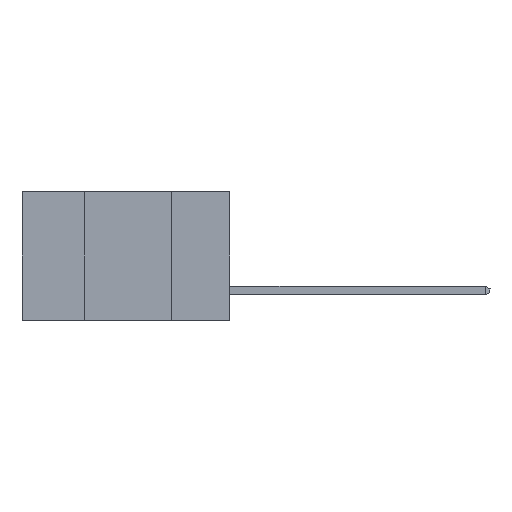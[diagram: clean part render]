
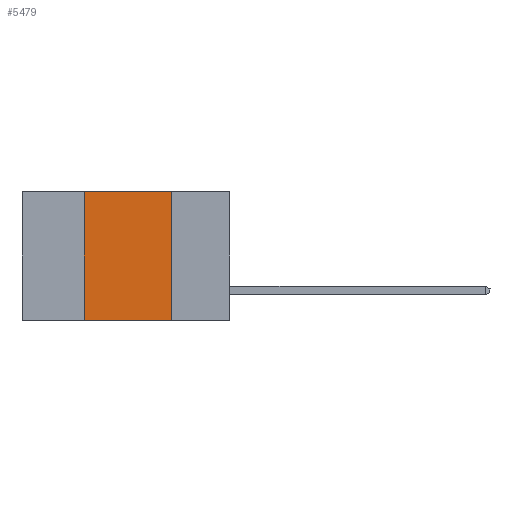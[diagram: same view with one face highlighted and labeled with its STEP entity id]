
A CAD part, left-side view. The second image highlights one B-rep face of the part: STEP entity #5479.
In plain terms, the highlighted planar face has unit normal (-1, 0, 0).
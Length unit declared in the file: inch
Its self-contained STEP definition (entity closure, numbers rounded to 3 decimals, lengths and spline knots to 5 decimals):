
#651 = VECTOR ( 'NONE', #3006, 39.37008 ) ;
#1235 = DIRECTION ( 'NONE',  ( 0., 0., -1. ) ) ;
#2057 = LINE ( 'NONE', #6154, #7532 ) ;
#2148 = DIRECTION ( 'NONE',  ( 0., 0., 1. ) ) ;
#2306 = CARTESIAN_POINT ( 'NONE',  ( 0., 0.42, -0.37 ) ) ;
#2531 = VERTEX_POINT ( 'NONE', #6071 ) ;
#2914 = CARTESIAN_POINT ( 'NONE',  ( 0., 0.17, -0.37 ) ) ;
#3006 = DIRECTION ( 'NONE',  ( 0., -1., 0. ) ) ;
#3350 = EDGE_CURVE ( 'NONE', #2531, #11595, #14398, .T. ) ;
#3627 = VECTOR ( 'NONE', #1235, 39.37008 ) ;
#4498 = VERTEX_POINT ( 'NONE', #2914 ) ;
#4834 = ORIENTED_EDGE ( 'NONE', *, *, #17452, .F. ) ;
#5479 = ADVANCED_FACE ( 'NONE', ( #7784 ), #17388, .F. ) ;
#6071 = CARTESIAN_POINT ( 'NONE',  ( 0., 0.42, 0. ) ) ;
#6154 = CARTESIAN_POINT ( 'NONE',  ( 0., 0.42, -0.37 ) ) ;
#6203 = DIRECTION ( 'NONE',  ( 1., 0., 0. ) ) ;
#6803 = ORIENTED_EDGE ( 'NONE', *, *, #15710, .T. ) ;
#6811 = AXIS2_PLACEMENT_3D ( 'NONE', #10497, #6203, #7614 ) ;
#7071 = EDGE_LOOP ( 'NONE', ( #17323, #12047, #4834, #6803 ) ) ;
#7104 = LINE ( 'NONE', #15414, #3627 ) ;
#7284 = EDGE_CURVE ( 'NONE', #11595, #4498, #7104, .T. ) ;
#7290 = CARTESIAN_POINT ( 'NONE',  ( 0., 0.6, -0.37 ) ) ;
#7532 = VECTOR ( 'NONE', #2148, 39.37008 ) ;
#7614 = DIRECTION ( 'NONE',  ( 0., 0., -1. ) ) ;
#7784 = FACE_OUTER_BOUND ( 'NONE', #7071, .T. ) ;
#8648 = CARTESIAN_POINT ( 'NONE',  ( 0., 0.17, 0. ) ) ;
#8693 = DIRECTION ( 'NONE',  ( 0., -1., 0. ) ) ;
#9198 = VECTOR ( 'NONE', #8693, 39.37008 ) ;
#9893 = VERTEX_POINT ( 'NONE', #2306 ) ;
#10193 = CARTESIAN_POINT ( 'NONE',  ( 0., 0.6, 0. ) ) ;
#10497 = CARTESIAN_POINT ( 'NONE',  ( 0., 0.6, 0. ) ) ;
#11595 = VERTEX_POINT ( 'NONE', #8648 ) ;
#12047 = ORIENTED_EDGE ( 'NONE', *, *, #3350, .F. ) ;
#12780 = LINE ( 'NONE', #7290, #651 ) ;
#14398 = LINE ( 'NONE', #10193, #9198 ) ;
#15414 = CARTESIAN_POINT ( 'NONE',  ( 0., 0.17, -0.37 ) ) ;
#15710 = EDGE_CURVE ( 'NONE', #9893, #4498, #12780, .T. ) ;
#17323 = ORIENTED_EDGE ( 'NONE', *, *, #7284, .F. ) ;
#17388 = PLANE ( 'NONE',  #6811 ) ;
#17452 = EDGE_CURVE ( 'NONE', #9893, #2531, #2057, .T. ) ;
